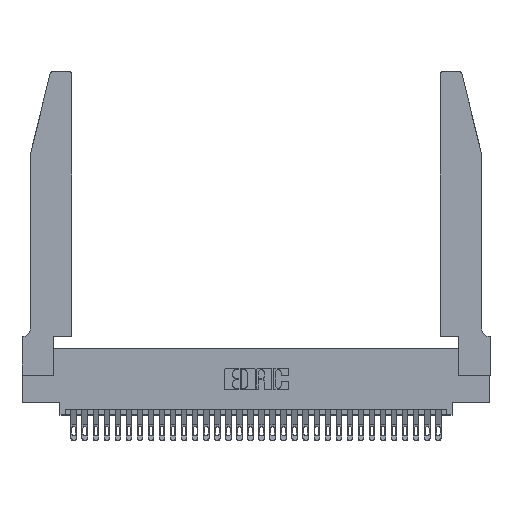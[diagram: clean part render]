
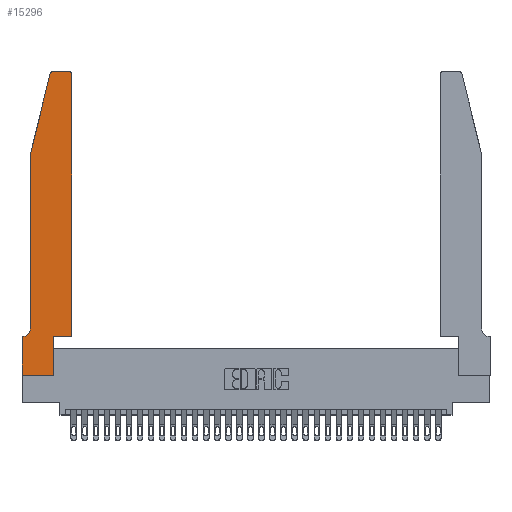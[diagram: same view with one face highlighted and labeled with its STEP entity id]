
A CAD part, top view. The second image highlights one B-rep face of the part: STEP entity #15296.
In plain terms, the highlighted planar face has unit normal (0, 0, 1).
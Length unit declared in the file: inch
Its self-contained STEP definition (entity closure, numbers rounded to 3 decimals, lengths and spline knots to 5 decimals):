
#19 = VERTEX_POINT ( 'NONE', #20607 ) ;
#30 = VECTOR ( 'NONE', #23603, 39.37008 ) ;
#331 = VERTEX_POINT ( 'NONE', #9030 ) ;
#391 = EDGE_CURVE ( 'NONE', #30944, #18196, #30068, .T. ) ;
#548 = CARTESIAN_POINT ( 'NONE',  ( 0.4505, 0.35, 0.37 ) ) ;
#1362 = EDGE_CURVE ( 'NONE', #20006, #26963, #24783, .T. ) ;
#2005 = AXIS2_PLACEMENT_3D ( 'NONE', #13322, #30820, #23133 ) ;
#2013 = EDGE_CURVE ( 'NONE', #26451, #30467, #8462, .T. ) ;
#2128 = CARTESIAN_POINT ( 'NONE',  ( 0.4205, 2.75, 0.37 ) ) ;
#2469 = VERTEX_POINT ( 'NONE', #9005 ) ;
#2828 = CARTESIAN_POINT ( 'NONE',  ( 0.4505, 0.35, 0.37 ) ) ;
#3226 = LINE ( 'NONE', #9881, #10801 ) ;
#3504 = CARTESIAN_POINT ( 'NONE',  ( 0.284, 2.72, 0.37 ) ) ;
#3803 = EDGE_CURVE ( 'NONE', #19, #26451, #30289, .T. ) ;
#3987 = EDGE_CURVE ( 'NONE', #16262, #11565, #31096, .T. ) ;
#4167 = DIRECTION ( 'NONE',  ( 0., 0., -1. ) ) ;
#6811 = CARTESIAN_POINT ( 'NONE',  ( 0.0055, 0.42, 0.37 ) ) ;
#6819 = DIRECTION ( 'NONE',  ( 1., 0., 0. ) ) ;
#6913 = ORIENTED_EDGE ( 'NONE', *, *, #31355, .T. ) ;
#7046 = DIRECTION ( 'NONE',  ( -1., 0., 0. ) ) ;
#7403 = VECTOR ( 'NONE', #7046, 39.37008 ) ;
#8365 = CARTESIAN_POINT ( 'NONE',  ( 0.2865, 0., 0.37 ) ) ;
#8400 = LINE ( 'NONE', #15779, #30 ) ;
#8462 = LINE ( 'NONE', #15086, #21215 ) ;
#9005 = CARTESIAN_POINT ( 'NONE',  ( 0., 0.35, 0.37 ) ) ;
#9030 = CARTESIAN_POINT ( 'NONE',  ( 0.0055, 0.35, 0.37 ) ) ;
#9250 = ORIENTED_EDGE ( 'NONE', *, *, #1362, .T. ) ;
#9726 = ORIENTED_EDGE ( 'NONE', *, *, #30317, .T. ) ;
#9881 = CARTESIAN_POINT ( 'NONE',  ( 0., 0., 0.37 ) ) ;
#10163 = EDGE_CURVE ( 'NONE', #2469, #16262, #3226, .T. ) ;
#10167 = EDGE_CURVE ( 'NONE', #30467, #27181, #12761, .T. ) ;
#10801 = VECTOR ( 'NONE', #22574, 39.37008 ) ;
#11090 = DIRECTION ( 'NONE',  ( 1., 0., 0. ) ) ;
#11565 = VERTEX_POINT ( 'NONE', #8365 ) ;
#11711 = CARTESIAN_POINT ( 'NONE',  ( 0.0755, 2., 0.37 ) ) ;
#11947 = AXIS2_PLACEMENT_3D ( 'NONE', #3504, #23885, #11090 ) ;
#11958 = PLANE ( 'NONE',  #14865 ) ;
#12043 = ORIENTED_EDGE ( 'NONE', *, *, #3987, .T. ) ;
#12049 = ORIENTED_EDGE ( 'NONE', *, *, #15814, .T. ) ;
#12761 = CIRCLE ( 'NONE', #2005, 0.03 ) ;
#13322 = CARTESIAN_POINT ( 'NONE',  ( 0.4205, 2.72, 0.37 ) ) ;
#13344 = DIRECTION ( 'NONE',  ( 1., 0., 0. ) ) ;
#14014 = CARTESIAN_POINT ( 'NONE',  ( 0.4505, 2.72, 0.37 ) ) ;
#14178 = LINE ( 'NONE', #14602, #7403 ) ;
#14602 = CARTESIAN_POINT ( 'NONE',  ( 0.0755, 0.35, 0.37 ) ) ;
#14865 = AXIS2_PLACEMENT_3D ( 'NONE', #32118, #29764, #6819 ) ;
#15086 = CARTESIAN_POINT ( 'NONE',  ( 0.4505, 0.35, 0.37 ) ) ;
#15296 = ADVANCED_FACE ( 'NONE', ( #18543 ), #11958, .T. ) ;
#15550 = CARTESIAN_POINT ( 'NONE',  ( 0., 0., 0.37 ) ) ;
#15779 = CARTESIAN_POINT ( 'NONE',  ( 0.2865, 0.35, 0.37 ) ) ;
#15814 = EDGE_CURVE ( 'NONE', #26963, #30944, #26081, .T. ) ;
#15820 = DIRECTION ( 'NONE',  ( -1., 0., 0. ) ) ;
#16262 = VERTEX_POINT ( 'NONE', #15550 ) ;
#16796 = DIRECTION ( 'NONE',  ( -0.239, -0.971, 0. ) ) ;
#17636 = ORIENTED_EDGE ( 'NONE', *, *, #2013, .T. ) ;
#18196 = VERTEX_POINT ( 'NONE', #32311 ) ;
#18509 = VECTOR ( 'NONE', #19368, 39.37008 ) ;
#18543 = FACE_OUTER_BOUND ( 'NONE', #21742, .T. ) ;
#19161 = CARTESIAN_POINT ( 'NONE',  ( 0.0755, 2., 0.37 ) ) ;
#19368 = DIRECTION ( 'NONE',  ( 0., -1., 0. ) ) ;
#20006 = VERTEX_POINT ( 'NONE', #26331 ) ;
#20025 = AXIS2_PLACEMENT_3D ( 'NONE', #6811, #4167, #27004 ) ;
#20280 = ORIENTED_EDGE ( 'NONE', *, *, #10167, .T. ) ;
#20367 = ORIENTED_EDGE ( 'NONE', *, *, #32983, .T. ) ;
#20607 = CARTESIAN_POINT ( 'NONE',  ( 0.2865, 0.35, 0.37 ) ) ;
#21215 = VECTOR ( 'NONE', #30593, 39.37008 ) ;
#21316 = CARTESIAN_POINT ( 'NONE',  ( 0.0755, 2., 0.37 ) ) ;
#21742 = EDGE_LOOP ( 'NONE', ( #6913, #9250, #12049, #22139, #24890, #20367, #24476, #12043, #9726, #30548, #17636, #20280 ) ) ;
#22002 = CARTESIAN_POINT ( 'NONE',  ( 0., 0., 0.37 ) ) ;
#22139 = ORIENTED_EDGE ( 'NONE', *, *, #391, .T. ) ;
#22574 = DIRECTION ( 'NONE',  ( 0., -1., 0. ) ) ;
#22712 = VECTOR ( 'NONE', #13344, 39.37008 ) ;
#23133 = DIRECTION ( 'NONE',  ( 1., 0., 0. ) ) ;
#23603 = DIRECTION ( 'NONE',  ( 0., 1., 0. ) ) ;
#23885 = DIRECTION ( 'NONE',  ( 0., 0., 1. ) ) ;
#24476 = ORIENTED_EDGE ( 'NONE', *, *, #10163, .T. ) ;
#24783 = CIRCLE ( 'NONE', #11947, 0.03 ) ;
#24890 = ORIENTED_EDGE ( 'NONE', *, *, #28862, .T. ) ;
#26081 = LINE ( 'NONE', #19161, #30423 ) ;
#26331 = CARTESIAN_POINT ( 'NONE',  ( 0.284, 2.75, 0.37 ) ) ;
#26451 = VERTEX_POINT ( 'NONE', #2828 ) ;
#26832 = DIRECTION ( 'NONE',  ( 1., 0., 0. ) ) ;
#26963 = VERTEX_POINT ( 'NONE', #27847 ) ;
#27004 = DIRECTION ( 'NONE',  ( -1., 0., 0. ) ) ;
#27060 = LINE ( 'NONE', #28324, #28233 ) ;
#27181 = VERTEX_POINT ( 'NONE', #2128 ) ;
#27619 = CIRCLE ( 'NONE', #20025, 0.07 ) ;
#27847 = CARTESIAN_POINT ( 'NONE',  ( 0.25487, 2.72718, 0.37 ) ) ;
#28233 = VECTOR ( 'NONE', #15820, 39.37008 ) ;
#28324 = CARTESIAN_POINT ( 'NONE',  ( 0.2605, 2.75, 0.37 ) ) ;
#28862 = EDGE_CURVE ( 'NONE', #18196, #331, #27619, .T. ) ;
#29764 = DIRECTION ( 'NONE',  ( 0., 0., 1. ) ) ;
#30068 = LINE ( 'NONE', #11711, #18509 ) ;
#30289 = LINE ( 'NONE', #548, #22712 ) ;
#30317 = EDGE_CURVE ( 'NONE', #11565, #19, #8400, .T. ) ;
#30423 = VECTOR ( 'NONE', #16796, 39.37008 ) ;
#30467 = VERTEX_POINT ( 'NONE', #14014 ) ;
#30548 = ORIENTED_EDGE ( 'NONE', *, *, #3803, .T. ) ;
#30593 = DIRECTION ( 'NONE',  ( 0., 1., 0. ) ) ;
#30820 = DIRECTION ( 'NONE',  ( 0., 0., 1. ) ) ;
#30944 = VERTEX_POINT ( 'NONE', #21316 ) ;
#31096 = LINE ( 'NONE', #22002, #31902 ) ;
#31355 = EDGE_CURVE ( 'NONE', #27181, #20006, #27060, .T. ) ;
#31902 = VECTOR ( 'NONE', #26832, 39.37008 ) ;
#32118 = CARTESIAN_POINT ( 'NONE',  ( 0., 0.35, 0.37 ) ) ;
#32311 = CARTESIAN_POINT ( 'NONE',  ( 0.0755, 0.42, 0.37 ) ) ;
#32983 = EDGE_CURVE ( 'NONE', #331, #2469, #14178, .T. ) ;
